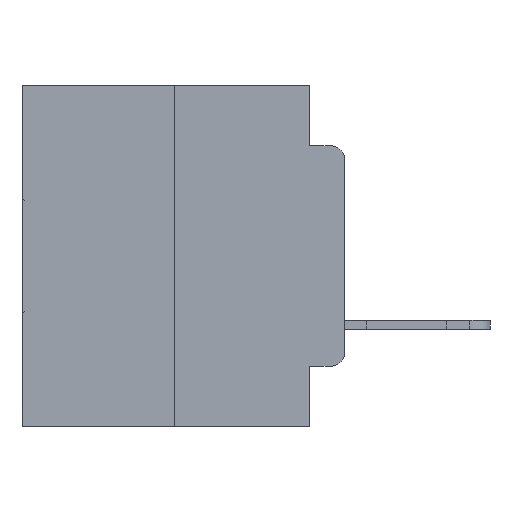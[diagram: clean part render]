
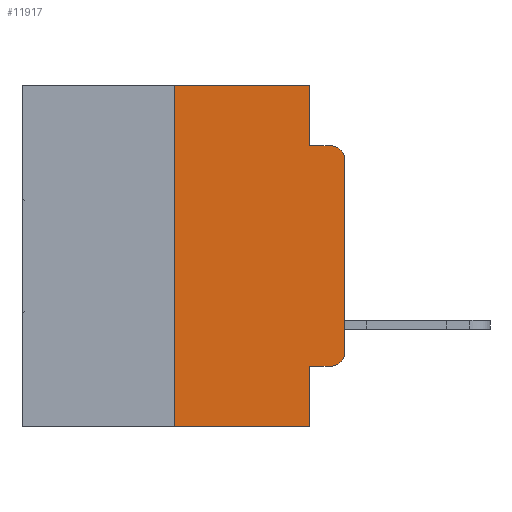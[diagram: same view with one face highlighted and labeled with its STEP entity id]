
A CAD part, left-side view. The second image highlights one B-rep face of the part: STEP entity #11917.
In plain terms, the highlighted planar face has unit normal (-1, 0, 0).
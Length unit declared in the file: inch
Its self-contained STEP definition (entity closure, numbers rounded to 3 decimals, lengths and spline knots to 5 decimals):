
#58 = CARTESIAN_POINT ( 'NONE',  ( 0., 0.02, -0.4115 ) ) ;
#573 = LINE ( 'NONE', #20693, #12184 ) ;
#2148 = LINE ( 'NONE', #26413, #14170 ) ;
#2206 = DIRECTION ( 'NONE',  ( 0., 0., -1. ) ) ;
#2297 = LINE ( 'NONE', #3545, #20137 ) ;
#2332 = DIRECTION ( 'NONE',  ( 1., 0., 0. ) ) ;
#2380 = LINE ( 'NONE', #3669, #14376 ) ;
#2644 = DIRECTION ( 'NONE',  ( 0., -1., 0. ) ) ;
#2814 = EDGE_CURVE ( 'NONE', #25427, #8153, #12959, .T. ) ;
#2852 = CARTESIAN_POINT ( 'NONE',  ( 0., 0.473, 0. ) ) ;
#3545 = CARTESIAN_POINT ( 'NONE',  ( 0., 0.25, 0. ) ) ;
#3628 = DIRECTION ( 'NONE',  ( 0., -1., 0. ) ) ;
#3643 = CARTESIAN_POINT ( 'NONE',  ( 0., 0.473, 0. ) ) ;
#3669 = CARTESIAN_POINT ( 'NONE',  ( 0., 0.051, -0.0885 ) ) ;
#3916 = EDGE_CURVE ( 'NONE', #23068, #16677, #14246, .T. ) ;
#3966 = VERTEX_POINT ( 'NONE', #16458 ) ;
#4489 = LINE ( 'NONE', #5286, #16109 ) ;
#4708 = DIRECTION ( 'NONE',  ( 0., 0., 1. ) ) ;
#4802 = EDGE_CURVE ( 'NONE', #10042, #3966, #2148, .T. ) ;
#5286 = CARTESIAN_POINT ( 'NONE',  ( 0., 0.051, -0.4115 ) ) ;
#5340 = PLANE ( 'NONE',  #14016 ) ;
#5817 = CARTESIAN_POINT ( 'NONE',  ( 0., 0., -0.1085 ) ) ;
#6771 = VERTEX_POINT ( 'NONE', #7484 ) ;
#7197 = VERTEX_POINT ( 'NONE', #17983 ) ;
#7256 = EDGE_CURVE ( 'NONE', #7197, #23068, #4489, .T. ) ;
#7379 = DIRECTION ( 'NONE',  ( 0., 0., 1. ) ) ;
#7389 = DIRECTION ( 'NONE',  ( 0., 0., -1. ) ) ;
#7408 = CARTESIAN_POINT ( 'NONE',  ( 0., 0.051, 0. ) ) ;
#7484 = CARTESIAN_POINT ( 'NONE',  ( 0., 0.02, -0.0885 ) ) ;
#8002 = ORIENTED_EDGE ( 'NONE', *, *, #28902, .T. ) ;
#8153 = VERTEX_POINT ( 'NONE', #8468 ) ;
#8294 = ORIENTED_EDGE ( 'NONE', *, *, #26353, .T. ) ;
#8385 = ORIENTED_EDGE ( 'NONE', *, *, #22250, .F. ) ;
#8468 = CARTESIAN_POINT ( 'NONE',  ( 0., 0.051, 0. ) ) ;
#8642 = ORIENTED_EDGE ( 'NONE', *, *, #17927, .F. ) ;
#8673 = ORIENTED_EDGE ( 'NONE', *, *, #2814, .F. ) ;
#8796 = EDGE_CURVE ( 'NONE', #7197, #3966, #573, .T. ) ;
#8903 = ORIENTED_EDGE ( 'NONE', *, *, #10313, .F. ) ;
#8983 = ORIENTED_EDGE ( 'NONE', *, *, #4802, .T. ) ;
#9210 = ORIENTED_EDGE ( 'NONE', *, *, #8796, .F. ) ;
#9385 = ORIENTED_EDGE ( 'NONE', *, *, #7256, .T. ) ;
#9461 = CARTESIAN_POINT ( 'NONE',  ( 0., 0.02, -0.1085 ) ) ;
#9467 = ORIENTED_EDGE ( 'NONE', *, *, #3916, .T. ) ;
#10042 = VERTEX_POINT ( 'NONE', #23716 ) ;
#10313 = EDGE_CURVE ( 'NONE', #10042, #25427, #2297, .T. ) ;
#11805 = DIRECTION ( 'NONE',  ( 0., 0., -1. ) ) ;
#11917 = ADVANCED_FACE ( 'NONE', ( #16332 ), #5340, .F. ) ;
#12184 = VECTOR ( 'NONE', #21728, 39.37008 ) ;
#12959 = LINE ( 'NONE', #3643, #27890 ) ;
#13166 = EDGE_LOOP ( 'NONE', ( #8002, #8294, #8385, #8642, #8673, #8903, #8983, #9210, #9385, #9467 ) ) ;
#13196 = VERTEX_POINT ( 'NONE', #15659 ) ;
#14016 = AXIS2_PLACEMENT_3D ( 'NONE', #2852, #2332, #2206 ) ;
#14170 = VECTOR ( 'NONE', #26366, 39.37008 ) ;
#14246 = CIRCLE ( 'NONE', #17424, 0.02 ) ;
#14376 = VECTOR ( 'NONE', #3628, 39.37008 ) ;
#15197 = CIRCLE ( 'NONE', #19111, 0.02 ) ;
#15659 = CARTESIAN_POINT ( 'NONE',  ( 0., 0.051, -0.0885 ) ) ;
#16046 = CARTESIAN_POINT ( 'NONE',  ( 0., 0.02, -0.3915 ) ) ;
#16109 = VECTOR ( 'NONE', #2644, 39.37008 ) ;
#16332 = FACE_OUTER_BOUND ( 'NONE', #13166, .T. ) ;
#16458 = CARTESIAN_POINT ( 'NONE',  ( 0., 0.051, -0.5 ) ) ;
#16535 = CARTESIAN_POINT ( 'NONE',  ( 0., 0.25, 0. ) ) ;
#16677 = VERTEX_POINT ( 'NONE', #26137 ) ;
#17424 = AXIS2_PLACEMENT_3D ( 'NONE', #16046, #18213, #23625 ) ;
#17674 = LINE ( 'NONE', #18664, #22677 ) ;
#17927 = EDGE_CURVE ( 'NONE', #8153, #13196, #18309, .T. ) ;
#17983 = CARTESIAN_POINT ( 'NONE',  ( 0., 0.051, -0.4115 ) ) ;
#18213 = DIRECTION ( 'NONE',  ( -1., 0., 0. ) ) ;
#18309 = LINE ( 'NONE', #7408, #22675 ) ;
#18664 = CARTESIAN_POINT ( 'NONE',  ( 0., 0., 0. ) ) ;
#19111 = AXIS2_PLACEMENT_3D ( 'NONE', #9461, #24830, #11805 ) ;
#20137 = VECTOR ( 'NONE', #4708, 39.37008 ) ;
#20693 = CARTESIAN_POINT ( 'NONE',  ( 0., 0.051, 0. ) ) ;
#21728 = DIRECTION ( 'NONE',  ( 0., 0., -1. ) ) ;
#22149 = DIRECTION ( 'NONE',  ( 0., -1., 0. ) ) ;
#22250 = EDGE_CURVE ( 'NONE', #13196, #6771, #2380, .T. ) ;
#22675 = VECTOR ( 'NONE', #7389, 39.37008 ) ;
#22677 = VECTOR ( 'NONE', #7379, 39.37008 ) ;
#23068 = VERTEX_POINT ( 'NONE', #58 ) ;
#23625 = DIRECTION ( 'NONE',  ( 0., 0., -1. ) ) ;
#23716 = CARTESIAN_POINT ( 'NONE',  ( 0., 0.25, -0.5 ) ) ;
#24830 = DIRECTION ( 'NONE',  ( -1., 0., 0. ) ) ;
#25427 = VERTEX_POINT ( 'NONE', #16535 ) ;
#26137 = CARTESIAN_POINT ( 'NONE',  ( 0., 0., -0.3915 ) ) ;
#26353 = EDGE_CURVE ( 'NONE', #27959, #6771, #15197, .T. ) ;
#26366 = DIRECTION ( 'NONE',  ( 0., -1., 0. ) ) ;
#26413 = CARTESIAN_POINT ( 'NONE',  ( 0., 0.473, -0.5 ) ) ;
#27890 = VECTOR ( 'NONE', #22149, 39.37008 ) ;
#27959 = VERTEX_POINT ( 'NONE', #5817 ) ;
#28902 = EDGE_CURVE ( 'NONE', #16677, #27959, #17674, .T. ) ;
